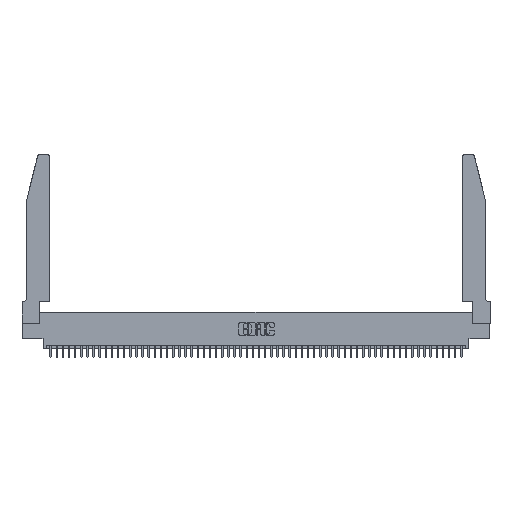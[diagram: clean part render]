
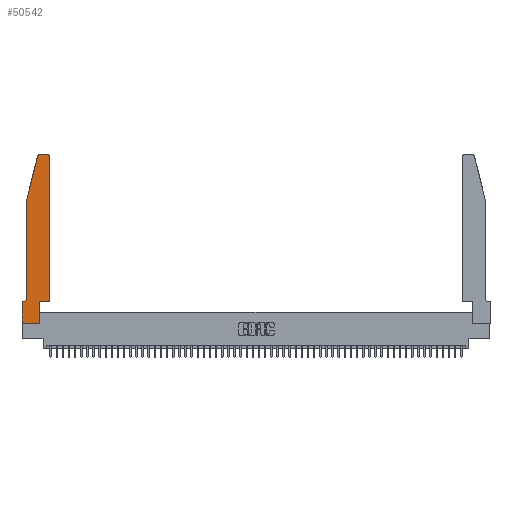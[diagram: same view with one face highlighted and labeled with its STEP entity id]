
A CAD part, top view. The second image highlights one B-rep face of the part: STEP entity #50542.
In plain terms, the highlighted planar face has unit normal (0, 0, 1).
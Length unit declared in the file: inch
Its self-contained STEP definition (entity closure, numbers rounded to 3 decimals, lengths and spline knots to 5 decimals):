
#197 = CIRCLE ( 'NONE', #44371, 0.07 ) ;
#430 = EDGE_CURVE ( 'NONE', #36342, #8427, #12155, .T. ) ;
#831 = ORIENTED_EDGE ( 'NONE', *, *, #37487, .T. ) ;
#1099 = CARTESIAN_POINT ( 'NONE',  ( 0., 0., 0.37 ) ) ;
#1683 = LINE ( 'NONE', #18170, #19578 ) ;
#2318 = ORIENTED_EDGE ( 'NONE', *, *, #43317, .T. ) ;
#2767 = EDGE_CURVE ( 'NONE', #19482, #26667, #31865, .T. ) ;
#2803 = CARTESIAN_POINT ( 'NONE',  ( 0.4505, 0.35, 0.37 ) ) ;
#3780 = DIRECTION ( 'NONE',  ( 1., 0., 0. ) ) ;
#4138 = CARTESIAN_POINT ( 'NONE',  ( 0.4505, 0.35, 0.37 ) ) ;
#4780 = DIRECTION ( 'NONE',  ( 1., 0., 0. ) ) ;
#4910 = CARTESIAN_POINT ( 'NONE',  ( 0.0755, 2., 0.37 ) ) ;
#5727 = DIRECTION ( 'NONE',  ( -0.239, -0.971, 0. ) ) ;
#5937 = VERTEX_POINT ( 'NONE', #33991 ) ;
#6126 = CARTESIAN_POINT ( 'NONE',  ( 0.4205, 2.75, 0.37 ) ) ;
#6939 = LINE ( 'NONE', #12014, #37391 ) ;
#7189 = CARTESIAN_POINT ( 'NONE',  ( 0.0055, 0.42, 0.37 ) ) ;
#7327 = ORIENTED_EDGE ( 'NONE', *, *, #21458, .T. ) ;
#7679 = CIRCLE ( 'NONE', #37905, 0.03 ) ;
#8427 = VERTEX_POINT ( 'NONE', #25903 ) ;
#9094 = VERTEX_POINT ( 'NONE', #4138 ) ;
#11759 = LINE ( 'NONE', #2803, #18481 ) ;
#11819 = EDGE_CURVE ( 'NONE', #15606, #12283, #47263, .T. ) ;
#12014 = CARTESIAN_POINT ( 'NONE',  ( 0.4505, 0.35, 0.37 ) ) ;
#12049 = CARTESIAN_POINT ( 'NONE',  ( 0.4205, 2.72, 0.37 ) ) ;
#12155 = LINE ( 'NONE', #31753, #28127 ) ;
#12283 = VERTEX_POINT ( 'NONE', #6126 ) ;
#12722 = VERTEX_POINT ( 'NONE', #34417 ) ;
#14973 = ORIENTED_EDGE ( 'NONE', *, *, #11819, .T. ) ;
#15072 = LINE ( 'NONE', #24523, #32280 ) ;
#15606 = VERTEX_POINT ( 'NONE', #27215 ) ;
#15734 = DIRECTION ( 'NONE',  ( 0., 0., -1. ) ) ;
#15835 = DIRECTION ( 'NONE',  ( 0., -1., 0. ) ) ;
#17171 = CARTESIAN_POINT ( 'NONE',  ( 0.0055, 0.35, 0.37 ) ) ;
#17451 = LINE ( 'NONE', #44894, #35341 ) ;
#18024 = EDGE_CURVE ( 'NONE', #5937, #46137, #7679, .T. ) ;
#18170 = CARTESIAN_POINT ( 'NONE',  ( 0.2865, 0.35, 0.37 ) ) ;
#18203 = ORIENTED_EDGE ( 'NONE', *, *, #33593, .T. ) ;
#18481 = VECTOR ( 'NONE', #23560, 39.37008 ) ;
#19313 = DIRECTION ( 'NONE',  ( 1., 0., 0. ) ) ;
#19325 = ORIENTED_EDGE ( 'NONE', *, *, #18024, .T. ) ;
#19482 = VERTEX_POINT ( 'NONE', #1099 ) ;
#19541 = DIRECTION ( 'NONE',  ( 0., 0., 1. ) ) ;
#19578 = VECTOR ( 'NONE', #51441, 39.37008 ) ;
#21458 = EDGE_CURVE ( 'NONE', #12722, #36342, #197, .T. ) ;
#22912 = DIRECTION ( 'NONE',  ( -1., 0., 0. ) ) ;
#23296 = ORIENTED_EDGE ( 'NONE', *, *, #51248, .T. ) ;
#23560 = DIRECTION ( 'NONE',  ( 0., 1., 0. ) ) ;
#24001 = DIRECTION ( 'NONE',  ( -1., 0., 0. ) ) ;
#24002 = FACE_OUTER_BOUND ( 'NONE', #49754, .T. ) ;
#24050 = CARTESIAN_POINT ( 'NONE',  ( 0.25487, 2.72718, 0.37 ) ) ;
#24523 = CARTESIAN_POINT ( 'NONE',  ( 0.0755, 2., 0.37 ) ) ;
#24687 = DIRECTION ( 'NONE',  ( 1., 0., 0. ) ) ;
#25103 = ORIENTED_EDGE ( 'NONE', *, *, #33989, .T. ) ;
#25267 = CARTESIAN_POINT ( 'NONE',  ( 0.284, 2.72, 0.37 ) ) ;
#25903 = CARTESIAN_POINT ( 'NONE',  ( 0., 0.35, 0.37 ) ) ;
#26667 = VERTEX_POINT ( 'NONE', #38283 ) ;
#27215 = CARTESIAN_POINT ( 'NONE',  ( 0.4505, 2.72, 0.37 ) ) ;
#27325 = ORIENTED_EDGE ( 'NONE', *, *, #42747, .T. ) ;
#27541 = DIRECTION ( 'NONE',  ( 1., 0., 0. ) ) ;
#28127 = VECTOR ( 'NONE', #22912, 39.37008 ) ;
#29276 = AXIS2_PLACEMENT_3D ( 'NONE', #12049, #32656, #24687 ) ;
#30772 = VECTOR ( 'NONE', #5727, 39.37008 ) ;
#30996 = ORIENTED_EDGE ( 'NONE', *, *, #33816, .T. ) ;
#31753 = CARTESIAN_POINT ( 'NONE',  ( 0.0755, 0.35, 0.37 ) ) ;
#31865 = LINE ( 'NONE', #46975, #53028 ) ;
#32280 = VECTOR ( 'NONE', #15835, 39.37008 ) ;
#32656 = DIRECTION ( 'NONE',  ( 0., 0., 1. ) ) ;
#32753 = DIRECTION ( 'NONE',  ( -1., 0., 0. ) ) ;
#33366 = ORIENTED_EDGE ( 'NONE', *, *, #430, .T. ) ;
#33593 = EDGE_CURVE ( 'NONE', #34013, #9094, #6939, .T. ) ;
#33816 = EDGE_CURVE ( 'NONE', #26667, #34013, #1683, .T. ) ;
#33989 = EDGE_CURVE ( 'NONE', #46137, #39363, #53250, .T. ) ;
#33991 = CARTESIAN_POINT ( 'NONE',  ( 0.284, 2.75, 0.37 ) ) ;
#34013 = VERTEX_POINT ( 'NONE', #43846 ) ;
#34417 = CARTESIAN_POINT ( 'NONE',  ( 0.0755, 0.42, 0.37 ) ) ;
#35341 = VECTOR ( 'NONE', #24001, 39.37008 ) ;
#36342 = VERTEX_POINT ( 'NONE', #17171 ) ;
#37249 = VECTOR ( 'NONE', #45034, 39.37008 ) ;
#37391 = VECTOR ( 'NONE', #19313, 39.37008 ) ;
#37487 = EDGE_CURVE ( 'NONE', #9094, #15606, #11759, .T. ) ;
#37905 = AXIS2_PLACEMENT_3D ( 'NONE', #25267, #54295, #3780 ) ;
#38283 = CARTESIAN_POINT ( 'NONE',  ( 0.2865, 0., 0.37 ) ) ;
#39363 = VERTEX_POINT ( 'NONE', #4910 ) ;
#42747 = EDGE_CURVE ( 'NONE', #12283, #5937, #17451, .T. ) ;
#43317 = EDGE_CURVE ( 'NONE', #8427, #19482, #53115, .T. ) ;
#43846 = CARTESIAN_POINT ( 'NONE',  ( 0.2865, 0.35, 0.37 ) ) ;
#44371 = AXIS2_PLACEMENT_3D ( 'NONE', #7189, #15734, #32753 ) ;
#44837 = CARTESIAN_POINT ( 'NONE',  ( 0., 0.35, 0.37 ) ) ;
#44894 = CARTESIAN_POINT ( 'NONE',  ( 0.2605, 2.75, 0.37 ) ) ;
#45034 = DIRECTION ( 'NONE',  ( 0., -1., 0. ) ) ;
#45199 = PLANE ( 'NONE',  #53844 ) ;
#46137 = VERTEX_POINT ( 'NONE', #24050 ) ;
#46975 = CARTESIAN_POINT ( 'NONE',  ( 0., 0., 0.37 ) ) ;
#47263 = CIRCLE ( 'NONE', #29276, 0.03 ) ;
#48962 = ORIENTED_EDGE ( 'NONE', *, *, #2767, .T. ) ;
#49754 = EDGE_LOOP ( 'NONE', ( #27325, #19325, #25103, #23296, #7327, #33366, #2318, #48962, #30996, #18203, #831, #14973 ) ) ;
#50542 = ADVANCED_FACE ( 'NONE', ( #24002 ), #45199, .T. ) ;
#51248 = EDGE_CURVE ( 'NONE', #39363, #12722, #15072, .T. ) ;
#51441 = DIRECTION ( 'NONE',  ( 0., 1., 0. ) ) ;
#52899 = CARTESIAN_POINT ( 'NONE',  ( 0.0755, 2., 0.37 ) ) ;
#53028 = VECTOR ( 'NONE', #4780, 39.37008 ) ;
#53115 = LINE ( 'NONE', #53191, #37249 ) ;
#53191 = CARTESIAN_POINT ( 'NONE',  ( 0., 0., 0.37 ) ) ;
#53250 = LINE ( 'NONE', #52899, #30772 ) ;
#53844 = AXIS2_PLACEMENT_3D ( 'NONE', #44837, #19541, #27541 ) ;
#54295 = DIRECTION ( 'NONE',  ( 0., 0., 1. ) ) ;
